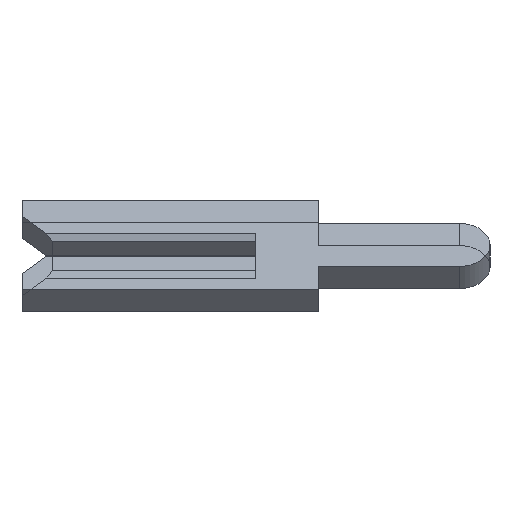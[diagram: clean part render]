
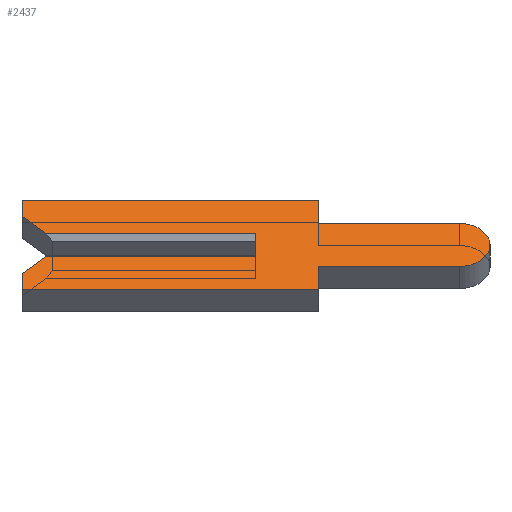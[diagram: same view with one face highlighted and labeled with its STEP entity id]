
A CAD part, left-side view. The second image highlights one B-rep face of the part: STEP entity #2437.
In plain terms, the highlighted face is planar.
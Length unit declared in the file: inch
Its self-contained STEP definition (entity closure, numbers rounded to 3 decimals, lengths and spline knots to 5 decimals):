
#22 = CARTESIAN_POINT ( 'NONE',  ( -0.01, 0.15, 0.026 ) ) ;
#40 = CARTESIAN_POINT ( 'NONE',  ( -0.01, -0.04, 0.0195 ) ) ;
#82 = EDGE_CURVE ( 'NONE', #3191, #2204, #2785, .T. ) ;
#88 = LINE ( 'NONE', #40, #2092 ) ;
#96 = CARTESIAN_POINT ( 'NONE',  ( -0.01, 0.15, 0.01 ) ) ;
#107 = CARTESIAN_POINT ( 'NONE',  ( -0.01, -0.04, 0.04 ) ) ;
#123 = VERTEX_POINT ( 'NONE', #827 ) ;
#165 = ORIENTED_EDGE ( 'NONE', *, *, #707, .F. ) ;
#173 = LINE ( 'NONE', #96, #2268 ) ;
#235 = ORIENTED_EDGE ( 'NONE', *, *, #82, .F. ) ;
#275 = CARTESIAN_POINT ( 'NONE',  ( -0.01, -0.04, -0.0195 ) ) ;
#283 = DIRECTION ( 'NONE',  ( 1., 0., 0. ) ) ;
#290 = ORIENTED_EDGE ( 'NONE', *, *, #2759, .F. ) ;
#307 = CARTESIAN_POINT ( 'NONE',  ( -0.01, 0.1305, 0.0065 ) ) ;
#313 = ORIENTED_EDGE ( 'NONE', *, *, #3403, .F. ) ;
#342 = CARTESIAN_POINT ( 'NONE',  ( -0.01, 0.15, -0.026 ) ) ;
#386 = VERTEX_POINT ( 'NONE', #275 ) ;
#397 = DIRECTION ( 'NONE',  ( 0., 0.707, 0.707 ) ) ;
#512 = DIRECTION ( 'NONE',  ( 1., 0., 0. ) ) ;
#610 = VERTEX_POINT ( 'NONE', #2770 ) ;
#659 = LINE ( 'NONE', #1493, #1577 ) ;
#690 = VERTEX_POINT ( 'NONE', #2962 ) ;
#704 = VECTOR ( 'NONE', #2465, 39.37008 ) ;
#707 = EDGE_CURVE ( 'NONE', #1346, #974, #1500, .T. ) ;
#721 = VECTOR ( 'NONE', #2327, 39.37008 ) ;
#745 = DIRECTION ( 'NONE',  ( 0., 0., -1. ) ) ;
#775 = CARTESIAN_POINT ( 'NONE',  ( -0.01, 0.15, 0.026 ) ) ;
#786 = LINE ( 'NONE', #1084, #2316 ) ;
#814 = EDGE_CURVE ( 'NONE', #123, #2732, #88, .T. ) ;
#827 = CARTESIAN_POINT ( 'NONE',  ( -0.01, -0.04, 0.0195 ) ) ;
#873 = LINE ( 'NONE', #2939, #3074 ) ;
#955 = CARTESIAN_POINT ( 'NONE',  ( -0.01, 0.15, -0.04 ) ) ;
#974 = VERTEX_POINT ( 'NONE', #342 ) ;
#985 = VERTEX_POINT ( 'NONE', #2515 ) ;
#1011 = LINE ( 'NONE', #2690, #1558 ) ;
#1042 = AXIS2_PLACEMENT_3D ( 'NONE', #1092, #283, #1646 ) ;
#1084 = CARTESIAN_POINT ( 'NONE',  ( -0.01, -0.1305, -0.01 ) ) ;
#1092 = CARTESIAN_POINT ( 'NONE',  ( -0.01, -0.1305, 0. ) ) ;
#1127 = DIRECTION ( 'NONE',  ( 0., -1., 0. ) ) ;
#1139 = EDGE_CURVE ( 'NONE', #974, #3098, #659, .T. ) ;
#1301 = DIRECTION ( 'NONE',  ( 0., 0., -1. ) ) ;
#1315 = EDGE_CURVE ( 'NONE', #3191, #3135, #173, .T. ) ;
#1342 = PLANE ( 'NONE',  #2279 ) ;
#1346 = VERTEX_POINT ( 'NONE', #955 ) ;
#1387 = EDGE_CURVE ( 'NONE', #386, #690, #1539, .T. ) ;
#1396 = DIRECTION ( 'NONE',  ( 0., 0., 1. ) ) ;
#1412 = CARTESIAN_POINT ( 'NONE',  ( -0.01, 0.15, -0.026 ) ) ;
#1462 = LINE ( 'NONE', #107, #2694 ) ;
#1482 = DIRECTION ( 'NONE',  ( 0., 0., -1. ) ) ;
#1493 = CARTESIAN_POINT ( 'NONE',  ( -0.01, 0.1305, -0.0065 ) ) ;
#1500 = LINE ( 'NONE', #1412, #1801 ) ;
#1502 = EDGE_CURVE ( 'NONE', #2339, #123, #1462, .T. ) ;
#1520 = LINE ( 'NONE', #3448, #721 ) ;
#1539 = LINE ( 'NONE', #2573, #2884 ) ;
#1543 = EDGE_CURVE ( 'NONE', #690, #1346, #1520, .T. ) ;
#1558 = VECTOR ( 'NONE', #1396, 39.37008 ) ;
#1564 = ORIENTED_EDGE ( 'NONE', *, *, #2935, .F. ) ;
#1577 = VECTOR ( 'NONE', #3076, 39.37008 ) ;
#1598 = CARTESIAN_POINT ( 'NONE',  ( -0.01, -0.1305, 0. ) ) ;
#1646 = DIRECTION ( 'NONE',  ( 0., 0., -1. ) ) ;
#1713 = ORIENTED_EDGE ( 'NONE', *, *, #1315, .T. ) ;
#1726 = FACE_OUTER_BOUND ( 'NONE', #2822, .T. ) ;
#1787 = VECTOR ( 'NONE', #397, 39.37008 ) ;
#1801 = VECTOR ( 'NONE', #3062, 39.37008 ) ;
#1819 = CARTESIAN_POINT ( 'NONE',  ( -0.01, -0.1305, -0.0195 ) ) ;
#1863 = CARTESIAN_POINT ( 'NONE',  ( -0.01, 0.15, 0.04 ) ) ;
#1877 = VERTEX_POINT ( 'NONE', #1819 ) ;
#1878 = CARTESIAN_POINT ( 'NONE',  ( -0.01, 0.134, 0.01 ) ) ;
#1988 = ORIENTED_EDGE ( 'NONE', *, *, #2154, .F. ) ;
#2034 = DIRECTION ( 'NONE',  ( 0., -1., 0. ) ) ;
#2092 = VECTOR ( 'NONE', #1127, 39.37008 ) ;
#2115 = ORIENTED_EDGE ( 'NONE', *, *, #1139, .F. ) ;
#2125 = CARTESIAN_POINT ( 'NONE',  ( -0.01, -0.1305, 0.0195 ) ) ;
#2142 = LINE ( 'NONE', #22, #704 ) ;
#2149 = DIRECTION ( 'NONE',  ( 0., -1., 0. ) ) ;
#2154 = EDGE_CURVE ( 'NONE', #610, #2339, #3048, .T. ) ;
#2204 = VERTEX_POINT ( 'NONE', #775 ) ;
#2268 = VECTOR ( 'NONE', #2034, 39.37008 ) ;
#2279 = AXIS2_PLACEMENT_3D ( 'NONE', #1598, #512, #1301 ) ;
#2316 = VECTOR ( 'NONE', #2149, 39.37008 ) ;
#2327 = DIRECTION ( 'NONE',  ( 0., 1., 0. ) ) ;
#2329 = ORIENTED_EDGE ( 'NONE', *, *, #3418, .F. ) ;
#2339 = VERTEX_POINT ( 'NONE', #2640 ) ;
#2365 = ORIENTED_EDGE ( 'NONE', *, *, #3363, .F. ) ;
#2377 = DIRECTION ( 'NONE',  ( 0., 1., 0. ) ) ;
#2403 = ORIENTED_EDGE ( 'NONE', *, *, #1502, .F. ) ;
#2437 = ADVANCED_FACE ( 'NONE', ( #1726 ), #1342, .F. ) ;
#2465 = DIRECTION ( 'NONE',  ( 0., 0., 1. ) ) ;
#2515 = CARTESIAN_POINT ( 'NONE',  ( -0.01, 0., -0.01 ) ) ;
#2573 = CARTESIAN_POINT ( 'NONE',  ( -0.01, -0.04, -0.04 ) ) ;
#2600 = VECTOR ( 'NONE', #3213, 39.37008 ) ;
#2640 = CARTESIAN_POINT ( 'NONE',  ( -0.01, -0.04, 0.04 ) ) ;
#2665 = ORIENTED_EDGE ( 'NONE', *, *, #814, .F. ) ;
#2682 = CARTESIAN_POINT ( 'NONE',  ( -0.01, 0., 0.01 ) ) ;
#2690 = CARTESIAN_POINT ( 'NONE',  ( -0.01, 0., 0.0065 ) ) ;
#2694 = VECTOR ( 'NONE', #745, 39.37008 ) ;
#2732 = VERTEX_POINT ( 'NONE', #2125 ) ;
#2742 = ORIENTED_EDGE ( 'NONE', *, *, #1543, .F. ) ;
#2759 = EDGE_CURVE ( 'NONE', #1877, #386, #873, .T. ) ;
#2770 = CARTESIAN_POINT ( 'NONE',  ( -0.01, 0.15, 0.04 ) ) ;
#2785 = LINE ( 'NONE', #307, #1787 ) ;
#2822 = EDGE_LOOP ( 'NONE', ( #1713, #2329, #1564, #2115, #165, #2742, #3108, #290, #2365, #2665, #2403, #1988, #313, #235 ) ) ;
#2884 = VECTOR ( 'NONE', #1482, 39.37008 ) ;
#2928 = CARTESIAN_POINT ( 'NONE',  ( -0.01, 0.134, -0.01 ) ) ;
#2935 = EDGE_CURVE ( 'NONE', #3098, #985, #786, .T. ) ;
#2939 = CARTESIAN_POINT ( 'NONE',  ( -0.01, -0.04, -0.0195 ) ) ;
#2962 = CARTESIAN_POINT ( 'NONE',  ( -0.01, -0.04, -0.04 ) ) ;
#3027 = CIRCLE ( 'NONE', #1042, 0.0195 ) ;
#3048 = LINE ( 'NONE', #1863, #2600 ) ;
#3062 = DIRECTION ( 'NONE',  ( 0., 0., 1. ) ) ;
#3074 = VECTOR ( 'NONE', #2377, 39.37008 ) ;
#3076 = DIRECTION ( 'NONE',  ( 0., -0.707, 0.707 ) ) ;
#3098 = VERTEX_POINT ( 'NONE', #2928 ) ;
#3108 = ORIENTED_EDGE ( 'NONE', *, *, #1387, .F. ) ;
#3135 = VERTEX_POINT ( 'NONE', #2682 ) ;
#3191 = VERTEX_POINT ( 'NONE', #1878 ) ;
#3213 = DIRECTION ( 'NONE',  ( 0., -1., 0. ) ) ;
#3363 = EDGE_CURVE ( 'NONE', #2732, #1877, #3027, .T. ) ;
#3403 = EDGE_CURVE ( 'NONE', #2204, #610, #2142, .T. ) ;
#3418 = EDGE_CURVE ( 'NONE', #985, #3135, #1011, .T. ) ;
#3448 = CARTESIAN_POINT ( 'NONE',  ( -0.01, 0.15, -0.04 ) ) ;
